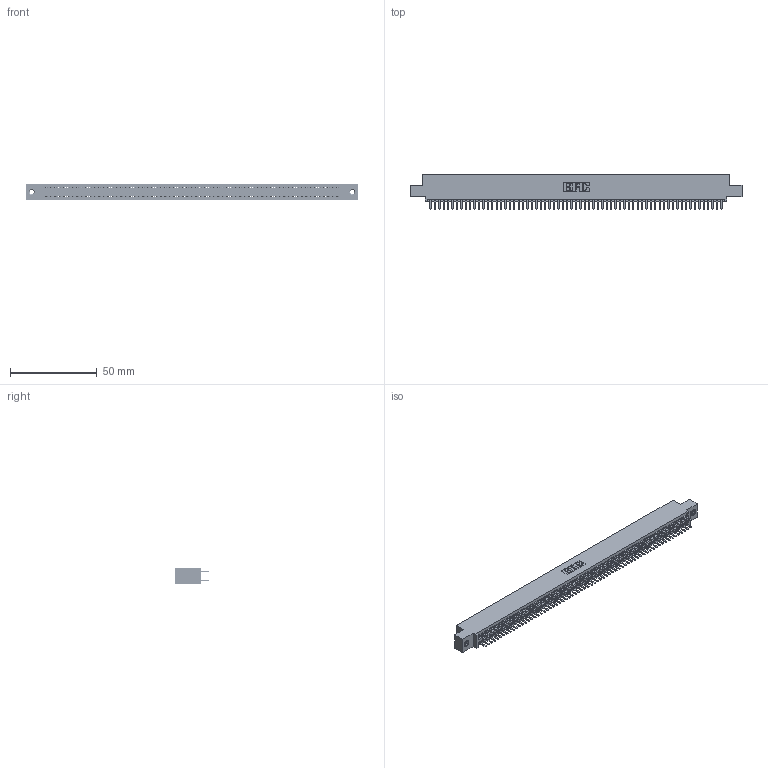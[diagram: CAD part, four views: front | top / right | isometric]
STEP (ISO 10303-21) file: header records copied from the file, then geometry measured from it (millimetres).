
FILE_DESCRIPTION (( 'STEP AP203' ), '1' );
FILE_NAME ('395-134-520-508.STEP', '2019-10-29T08:43:36', ( '' ), ( '' ), 'SwSTEP 2.0', 'SolidWorks 2016', '' );
FILE_SCHEMA (( 'CONFIG_CONTROL_DESIGN' ));
Length unit declared in the file: inch
Products named in the file (4): 345-292-001_345-293-120; 345-250-001_345-250-003-102; 395-134-520-508; 345 Part_0.110 Offset - 0.156 Dia-TI
Assembly tree (137 placements, depth 2):
  395-134-520-508
    345 Part_0.110 Offset - 0.156 Dia-TI
    345-292-001_345-293-120  x134
    345-250-001_345-250-003-102  x2
Bounding box: 191.39 x 19.68 x 9.4 mm (x, y, z)
Volume: 18685 mm3; surface area: 28084.7 mm2
Topology: 137 solids, 137 shells, 7426 faces, 21527 edges, 13986 vertices
Faces by surface type: plane 4806, cylinder 2604, cone 12, torus 4
Entity records: 50636 total; most frequent: CARTESIAN_POINT 8459, ORIENTED_EDGE 8374, DIRECTION 7441, EDGE_CURVE 4187, VECTOR 3763, LINE 3763, VERTEX_POINT 2784, AXIS2_PLACEMENT_3D 1839
